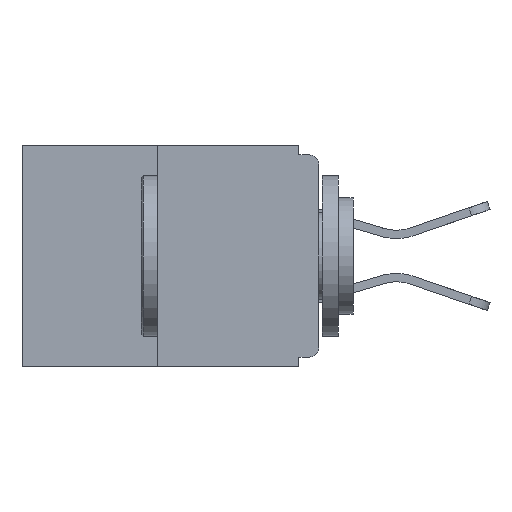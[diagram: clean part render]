
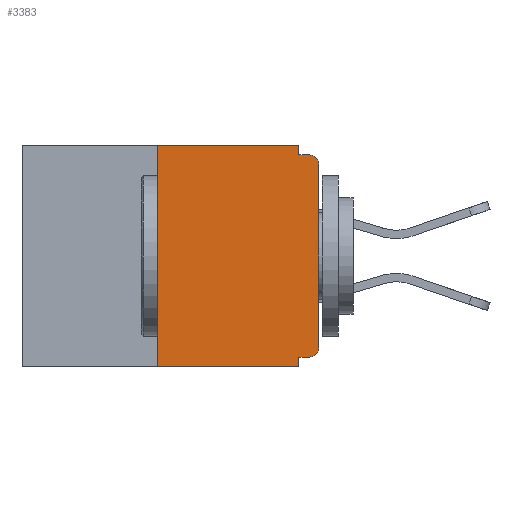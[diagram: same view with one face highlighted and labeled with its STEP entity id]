
A CAD part, left-side view. The second image highlights one B-rep face of the part: STEP entity #3383.
In plain terms, the highlighted planar face has unit normal (-1, 0, 0).
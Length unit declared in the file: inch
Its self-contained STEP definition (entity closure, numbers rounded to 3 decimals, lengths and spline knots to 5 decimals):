
#363 = DIRECTION ( 'NONE',  ( 0., 0., -1. ) ) ;
#748 = LINE ( 'NONE', #22695, #23737 ) ;
#752 = CARTESIAN_POINT ( 'NONE',  ( 0., 0.015, -0.313 ) ) ;
#876 = CARTESIAN_POINT ( 'NONE',  ( 0., 0., -0.03 ) ) ;
#1176 = FACE_OUTER_BOUND ( 'NONE', #20992, .T. ) ;
#1238 = CARTESIAN_POINT ( 'NONE',  ( 0., 0.031, 0. ) ) ;
#1371 = ORIENTED_EDGE ( 'NONE', *, *, #28385, .F. ) ;
#1912 = VERTEX_POINT ( 'NONE', #12458 ) ;
#2106 = CARTESIAN_POINT ( 'NONE',  ( 0., 0.031, -0.015 ) ) ;
#2489 = LINE ( 'NONE', #18281, #15729 ) ;
#3139 = EDGE_CURVE ( 'NONE', #27718, #16256, #11704, .T. ) ;
#3249 = EDGE_CURVE ( 'NONE', #10708, #16100, #15813, .T. ) ;
#3267 = DIRECTION ( 'NONE',  ( 0., 0., -1. ) ) ;
#3383 = ADVANCED_FACE ( 'NONE', ( #1176 ), #23999, .F. ) ;
#3385 = CIRCLE ( 'NONE', #5701, 0.015 ) ;
#5090 = ORIENTED_EDGE ( 'NONE', *, *, #21015, .T. ) ;
#5225 = EDGE_CURVE ( 'NONE', #16100, #8143, #748, .T. ) ;
#5701 = AXIS2_PLACEMENT_3D ( 'NONE', #13712, #11601, #26874 ) ;
#6169 = DIRECTION ( 'NONE',  ( 0., 0., -1. ) ) ;
#6425 = CARTESIAN_POINT ( 'NONE',  ( 0., 0.031, -0.328 ) ) ;
#7076 = CARTESIAN_POINT ( 'NONE',  ( 0., 0.031, 0. ) ) ;
#7551 = EDGE_CURVE ( 'NONE', #26246, #18446, #7943, .T. ) ;
#7603 = VECTOR ( 'NONE', #363, 39.37008 ) ;
#7737 = VECTOR ( 'NONE', #14122, 39.37008 ) ;
#7943 = LINE ( 'NONE', #22669, #7603 ) ;
#8143 = VERTEX_POINT ( 'NONE', #1238 ) ;
#9399 = EDGE_CURVE ( 'NONE', #25293, #1912, #3385, .T. ) ;
#10708 = VERTEX_POINT ( 'NONE', #26935 ) ;
#11287 = ORIENTED_EDGE ( 'NONE', *, *, #9399, .T. ) ;
#11601 = DIRECTION ( 'NONE',  ( -1., 0., 0. ) ) ;
#11704 = CIRCLE ( 'NONE', #19000, 0.015 ) ;
#11910 = DIRECTION ( 'NONE',  ( 0., -1., 0. ) ) ;
#11967 = VECTOR ( 'NONE', #20777, 39.37008 ) ;
#12387 = LINE ( 'NONE', #26986, #18258 ) ;
#12458 = CARTESIAN_POINT ( 'NONE',  ( 0., 0.015, -0.015 ) ) ;
#12717 = VECTOR ( 'NONE', #18918, 39.37008 ) ;
#12893 = AXIS2_PLACEMENT_3D ( 'NONE', #23902, #12921, #6169 ) ;
#12921 = DIRECTION ( 'NONE',  ( 1., 0., 0. ) ) ;
#13216 = ORIENTED_EDGE ( 'NONE', *, *, #28887, .F. ) ;
#13561 = ORIENTED_EDGE ( 'NONE', *, *, #7551, .F. ) ;
#13712 = CARTESIAN_POINT ( 'NONE',  ( 0., 0.015, -0.03 ) ) ;
#14122 = DIRECTION ( 'NONE',  ( 0., -1., 0. ) ) ;
#14270 = DIRECTION ( 'NONE',  ( -1., 0., 0. ) ) ;
#14745 = VECTOR ( 'NONE', #22617, 39.37008 ) ;
#15178 = CARTESIAN_POINT ( 'NONE',  ( 0., 0.015, -0.328 ) ) ;
#15729 = VECTOR ( 'NONE', #11910, 39.37008 ) ;
#15813 = LINE ( 'NONE', #23527, #12717 ) ;
#15840 = CARTESIAN_POINT ( 'NONE',  ( 0., 0.25, 0. ) ) ;
#16100 = VERTEX_POINT ( 'NONE', #15840 ) ;
#16256 = VERTEX_POINT ( 'NONE', #24638 ) ;
#16442 = EDGE_CURVE ( 'NONE', #10708, #18446, #2489, .T. ) ;
#16669 = VERTEX_POINT ( 'NONE', #2106 ) ;
#17208 = ORIENTED_EDGE ( 'NONE', *, *, #26477, .F. ) ;
#18258 = VECTOR ( 'NONE', #20107, 39.37008 ) ;
#18281 = CARTESIAN_POINT ( 'NONE',  ( 0., 0.46, -0.343 ) ) ;
#18381 = CARTESIAN_POINT ( 'NONE',  ( 0., 0., -0.015 ) ) ;
#18446 = VERTEX_POINT ( 'NONE', #25477 ) ;
#18492 = LINE ( 'NONE', #18381, #7737 ) ;
#18918 = DIRECTION ( 'NONE',  ( 0., 0., 1. ) ) ;
#19000 = AXIS2_PLACEMENT_3D ( 'NONE', #752, #14270, #3267 ) ;
#19997 = ORIENTED_EDGE ( 'NONE', *, *, #16442, .T. ) ;
#20107 = DIRECTION ( 'NONE',  ( 0., 0., 1. ) ) ;
#20650 = LINE ( 'NONE', #22524, #14745 ) ;
#20777 = DIRECTION ( 'NONE',  ( 0., 0., -1. ) ) ;
#20992 = EDGE_LOOP ( 'NONE', ( #23923, #27319, #19997, #13561, #17208, #25098, #5090, #11287, #13216, #1371 ) ) ;
#21015 = EDGE_CURVE ( 'NONE', #16256, #25293, #12387, .T. ) ;
#22524 = CARTESIAN_POINT ( 'NONE',  ( 0., 0., -0.328 ) ) ;
#22617 = DIRECTION ( 'NONE',  ( 0., 1., 0. ) ) ;
#22669 = CARTESIAN_POINT ( 'NONE',  ( 0., 0.031, -0.343 ) ) ;
#22695 = CARTESIAN_POINT ( 'NONE',  ( 0., 0.46, 0. ) ) ;
#23527 = CARTESIAN_POINT ( 'NONE',  ( 0., 0.25, 0. ) ) ;
#23737 = VECTOR ( 'NONE', #26917, 39.37008 ) ;
#23902 = CARTESIAN_POINT ( 'NONE',  ( 0., 0.46, 0. ) ) ;
#23923 = ORIENTED_EDGE ( 'NONE', *, *, #5225, .F. ) ;
#23999 = PLANE ( 'NONE',  #12893 ) ;
#24638 = CARTESIAN_POINT ( 'NONE',  ( 0., 0., -0.313 ) ) ;
#25098 = ORIENTED_EDGE ( 'NONE', *, *, #3139, .T. ) ;
#25293 = VERTEX_POINT ( 'NONE', #876 ) ;
#25477 = CARTESIAN_POINT ( 'NONE',  ( 0., 0.031, -0.343 ) ) ;
#26246 = VERTEX_POINT ( 'NONE', #6425 ) ;
#26477 = EDGE_CURVE ( 'NONE', #27718, #26246, #20650, .T. ) ;
#26874 = DIRECTION ( 'NONE',  ( 0., 0., -1. ) ) ;
#26917 = DIRECTION ( 'NONE',  ( 0., -1., 0. ) ) ;
#26935 = CARTESIAN_POINT ( 'NONE',  ( 0., 0.25, -0.343 ) ) ;
#26986 = CARTESIAN_POINT ( 'NONE',  ( 0., 0., 0. ) ) ;
#27319 = ORIENTED_EDGE ( 'NONE', *, *, #3249, .F. ) ;
#27718 = VERTEX_POINT ( 'NONE', #15178 ) ;
#28335 = LINE ( 'NONE', #7076, #11967 ) ;
#28385 = EDGE_CURVE ( 'NONE', #8143, #16669, #28335, .T. ) ;
#28887 = EDGE_CURVE ( 'NONE', #16669, #1912, #18492, .T. ) ;
